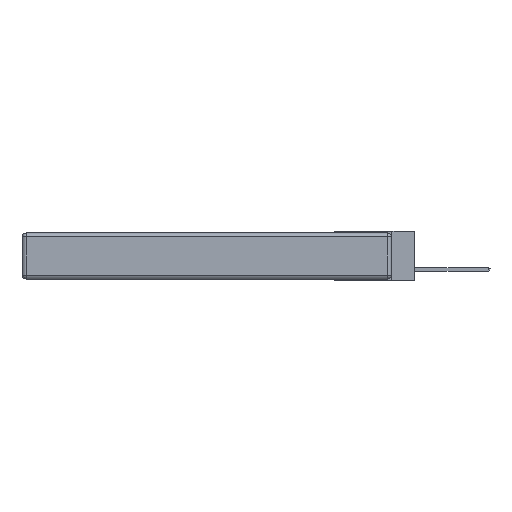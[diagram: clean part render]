
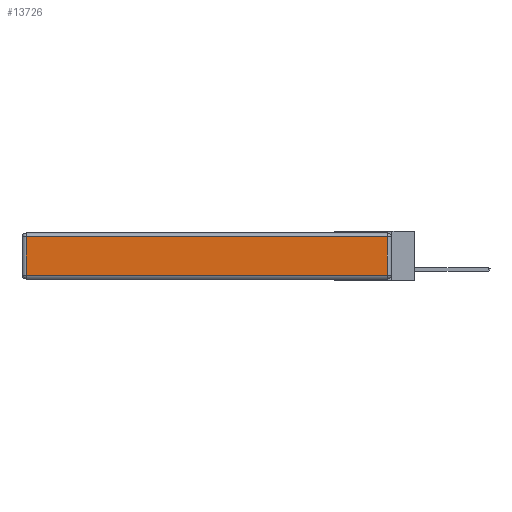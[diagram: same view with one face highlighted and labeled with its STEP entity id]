
A CAD part, left-side view. The second image highlights one B-rep face of the part: STEP entity #13726.
In plain terms, the highlighted planar face has unit normal (-1, 0, 0).
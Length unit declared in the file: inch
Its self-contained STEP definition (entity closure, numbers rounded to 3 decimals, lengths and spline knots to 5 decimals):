
#153 = CARTESIAN_POINT ( 'NONE',  ( 0., 0.03, -0.313 ) ) ;
#286 = DIRECTION ( 'NONE',  ( 0., 0., 1. ) ) ;
#471 = DIRECTION ( 'NONE',  ( 0., 0., -1. ) ) ;
#644 = LINE ( 'NONE', #33051, #16590 ) ;
#672 = LINE ( 'NONE', #14585, #27871 ) ;
#859 = LINE ( 'NONE', #7233, #31453 ) ;
#1327 = CARTESIAN_POINT ( 'NONE',  ( 0., 0.03, -0.03 ) ) ;
#1544 = VECTOR ( 'NONE', #30490, 39.37008 ) ;
#5412 = EDGE_CURVE ( 'NONE', #27731, #27593, #31325, .T. ) ;
#5452 = CARTESIAN_POINT ( 'NONE',  ( 0., 0., -0.343 ) ) ;
#5819 = CARTESIAN_POINT ( 'NONE',  ( 0., 2.72, -0.03 ) ) ;
#6689 = VERTEX_POINT ( 'NONE', #1327 ) ;
#7233 = CARTESIAN_POINT ( 'NONE',  ( 0., 0.03, -0.343 ) ) ;
#10967 = PLANE ( 'NONE',  #15117 ) ;
#11117 = VERTEX_POINT ( 'NONE', #5819 ) ;
#11761 = CARTESIAN_POINT ( 'NONE',  ( 0., 0., -0.313 ) ) ;
#11842 = EDGE_CURVE ( 'NONE', #11117, #27731, #644, .T. ) ;
#13671 = EDGE_LOOP ( 'NONE', ( #14437, #31242, #27135, #17513 ) ) ;
#13726 = ADVANCED_FACE ( 'NONE', ( #21470 ), #10967, .T. ) ;
#14437 = ORIENTED_EDGE ( 'NONE', *, *, #5412, .T. ) ;
#14585 = CARTESIAN_POINT ( 'NONE',  ( 0., 2.75, -0.03 ) ) ;
#15117 = AXIS2_PLACEMENT_3D ( 'NONE', #5452, #18717, #286 ) ;
#16590 = VECTOR ( 'NONE', #471, 39.37008 ) ;
#17513 = ORIENTED_EDGE ( 'NONE', *, *, #11842, .T. ) ;
#18717 = DIRECTION ( 'NONE',  ( -1., 0., 0. ) ) ;
#21470 = FACE_OUTER_BOUND ( 'NONE', #13671, .T. ) ;
#26962 = EDGE_CURVE ( 'NONE', #27593, #6689, #859, .T. ) ;
#27135 = ORIENTED_EDGE ( 'NONE', *, *, #28474, .T. ) ;
#27593 = VERTEX_POINT ( 'NONE', #153 ) ;
#27731 = VERTEX_POINT ( 'NONE', #33197 ) ;
#27871 = VECTOR ( 'NONE', #30426, 39.37008 ) ;
#28474 = EDGE_CURVE ( 'NONE', #6689, #11117, #672, .T. ) ;
#30426 = DIRECTION ( 'NONE',  ( 0., 1., 0. ) ) ;
#30490 = DIRECTION ( 'NONE',  ( 0., -1., 0. ) ) ;
#31242 = ORIENTED_EDGE ( 'NONE', *, *, #26962, .T. ) ;
#31325 = LINE ( 'NONE', #11761, #1544 ) ;
#31453 = VECTOR ( 'NONE', #34302, 39.37008 ) ;
#33051 = CARTESIAN_POINT ( 'NONE',  ( 0., 2.72, -0.343 ) ) ;
#33197 = CARTESIAN_POINT ( 'NONE',  ( 0., 2.72, -0.313 ) ) ;
#34302 = DIRECTION ( 'NONE',  ( 0., 0., 1. ) ) ;
